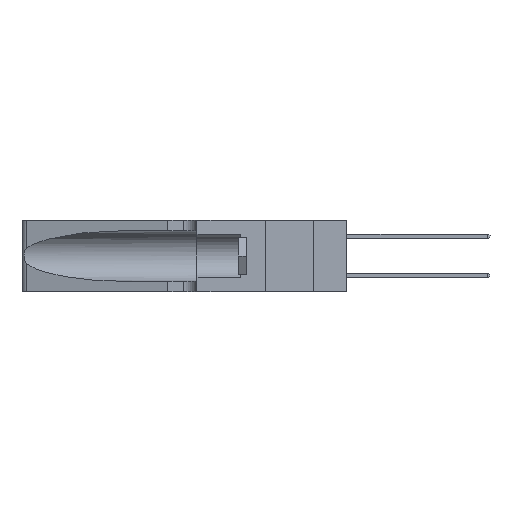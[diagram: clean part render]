
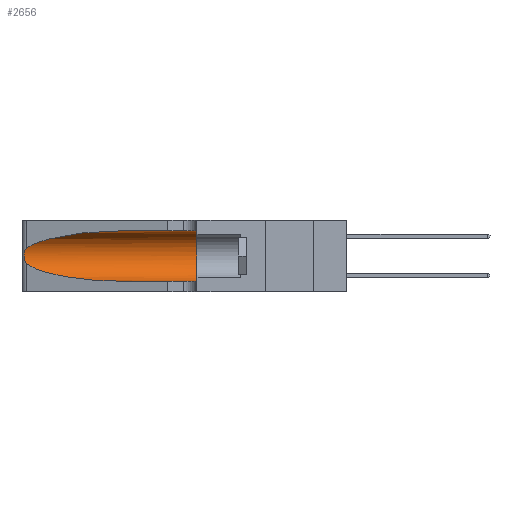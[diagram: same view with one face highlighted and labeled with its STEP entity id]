
A CAD part, left-side view. The second image highlights one B-rep face of the part: STEP entity #2656.
In plain terms, the highlighted cylindrical face has radius 3.308 mm (diameter 6.617 mm), a partial arc.
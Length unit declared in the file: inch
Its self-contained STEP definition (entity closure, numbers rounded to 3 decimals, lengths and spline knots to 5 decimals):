
#344 = VECTOR ( 'NONE', #13298, 39.37008 ) ;
#855 = CIRCLE ( 'NONE', #21152, 0.13025 ) ;
#1330 = DIRECTION ( 'NONE',  ( 0., -1., 0. ) ) ;
#1814 = CARTESIAN_POINT ( 'NONE',  ( 0.1305, 1.61858, 0.05475 ) ) ;
#1860 = DIRECTION ( 'NONE',  ( 0., 1., 0. ) ) ;
#2656 = ADVANCED_FACE ( 'NONE', ( #17979 ), #35239, .F. ) ;
#2858 = VECTOR ( 'NONE', #27332, 39.37008 ) ;
#2972 = VERTEX_POINT ( 'NONE', #34383 ) ;
#3401 = CARTESIAN_POINT ( 'NONE',  ( 0.25487, 1.22718, 0.14631 ) ) ;
#3728 = CARTESIAN_POINT ( 'NONE',  ( 0.18966, 0.96281, 0.31525 ) ) ;
#3752 = CARTESIAN_POINT ( 'NONE',  ( 0.2373, 1.15595, 0.08982 ) ) ;
#4124 = VERTEX_POINT ( 'NONE', #12017 ) ;
#4175 = EDGE_CURVE ( 'NONE', #15163, #4124, #11915, .T. ) ;
#4205 = CARTESIAN_POINT ( 'NONE',  ( 0.25854, 1.2359, 0.20912 ) ) ;
#4450 = ORIENTED_EDGE ( 'NONE', *, *, #34418, .F. ) ;
#6496 = CARTESIAN_POINT ( 'NONE',  ( 0.2373, 1.15595, 0.28018 ) ) ;
#7114 = CARTESIAN_POINT ( 'NONE',  ( 0.18966, 0.96281, 0.05475 ) ) ;
#7706 = EDGE_LOOP ( 'NONE', ( #17933, #35705, #15451, #27042, #4450, #12828 ) ) ;
#7805 = EDGE_CURVE ( 'NONE', #33567, #8279, #21128, .T. ) ;
#8279 = VERTEX_POINT ( 'NONE', #16266 ) ;
#9377 = EDGE_CURVE ( 'NONE', #2972, #33567, #30256, .T. ) ;
#11073 = AXIS2_PLACEMENT_3D ( 'NONE', #20027, #1330, #31758 ) ;
#11915 = LINE ( 'NONE', #25645, #2858 ) ;
#12017 = CARTESIAN_POINT ( 'NONE',  ( 0.1305, 0.35, 0.31525 ) ) ;
#12051 = CARTESIAN_POINT ( 'NONE',  ( 0.26018, 1.23835, 0.19895 ) ) ;
#12190 = CARTESIAN_POINT ( 'NONE',  ( 0.25487, 1.22718, 0.14631 ) ) ;
#12828 = ORIENTED_EDGE ( 'NONE', *, *, #4175, .F. ) ;
#13298 = DIRECTION ( 'NONE',  ( 0., -1., 0. ) ) ;
#13360 = CARTESIAN_POINT ( 'NONE',  ( 0.25555, 1.22993, 0.14849 ) ) ;
#13477 = DIRECTION ( 'NONE',  ( 0., 0., 1. ) ) ;
#14218 = CARTESIAN_POINT ( 'NONE',  ( 0.25487, 1.22718, 0.22369 ) ) ;
#14341 = CARTESIAN_POINT ( 'NONE',  ( 0.25555, 1.22994, 0.2215 ) ) ;
#15117 = EDGE_CURVE ( 'NONE', #15163, #2972, #15892, .T. ) ;
#15163 = VERTEX_POINT ( 'NONE', #28857 ) ;
#15451 = ORIENTED_EDGE ( 'NONE', *, *, #7805, .T. ) ;
#15892 =( BOUNDED_CURVE ( )  B_SPLINE_CURVE ( 3, ( #30749, #3728, #6496, #25653 ),
 .UNSPECIFIED., .F., .F. ) 
 B_SPLINE_CURVE_WITH_KNOTS ( ( 4, 4 ),
 ( 1.5708, 2.84003 ),
 .UNSPECIFIED. ) 
 CURVE ( )  GEOMETRIC_REPRESENTATION_ITEM ( )  RATIONAL_B_SPLINE_CURVE ( ( 1., 0.87, 0.87, 1. ) ) 
 REPRESENTATION_ITEM ( '' )  );
#15898 = CARTESIAN_POINT ( 'NONE',  ( 0.25856, 1.23593, 0.16098 ) ) ;
#16018 = CARTESIAN_POINT ( 'NONE',  ( 0.25639, 1.23186, 0.15144 ) ) ;
#16266 = CARTESIAN_POINT ( 'NONE',  ( 0.1305, 0.72297, 0.05475 ) ) ;
#17693 = CARTESIAN_POINT ( 'NONE',  ( 0.25639, 1.23184, 0.21858 ) ) ;
#17933 = ORIENTED_EDGE ( 'NONE', *, *, #15117, .T. ) ;
#17979 = FACE_OUTER_BOUND ( 'NONE', #7706, .T. ) ;
#18773 = CARTESIAN_POINT ( 'NONE',  ( 0.1305, 0.35, 0.185 ) ) ;
#20027 = CARTESIAN_POINT ( 'NONE',  ( 0.1305, 1.61858, 0.185 ) ) ;
#21128 =( BOUNDED_CURVE ( )  B_SPLINE_CURVE ( 3, ( #3401, #3752, #7114, #29048 ),
 .UNSPECIFIED., .F., .F. ) 
 B_SPLINE_CURVE_WITH_KNOTS ( ( 4, 4 ),
 ( 3.44316, 4.71239 ),
 .UNSPECIFIED. ) 
 CURVE ( )  GEOMETRIC_REPRESENTATION_ITEM ( )  RATIONAL_B_SPLINE_CURVE ( ( 1., 0.87, 0.87, 1. ) ) 
 REPRESENTATION_ITEM ( '' )  );
#21152 = AXIS2_PLACEMENT_3D ( 'NONE', #18773, #1860, #13477 ) ;
#24091 = CARTESIAN_POINT ( 'NONE',  ( 0.26017, 1.23833, 0.17102 ) ) ;
#25645 = CARTESIAN_POINT ( 'NONE',  ( 0.1305, 1.61858, 0.31525 ) ) ;
#25653 = CARTESIAN_POINT ( 'NONE',  ( 0.25487, 1.22718, 0.22369 ) ) ;
#27042 = ORIENTED_EDGE ( 'NONE', *, *, #31643, .T. ) ;
#27215 = CARTESIAN_POINT ( 'NONE',  ( 0.25789, 1.23486, 0.15765 ) ) ;
#27332 = DIRECTION ( 'NONE',  ( 0., -1., 0. ) ) ;
#28551 = CARTESIAN_POINT ( 'NONE',  ( 0.25787, 1.23484, 0.2124 ) ) ;
#28702 = VERTEX_POINT ( 'NONE', #30568 ) ;
#28857 = CARTESIAN_POINT ( 'NONE',  ( 0.1305, 0.72297, 0.31525 ) ) ;
#29048 = CARTESIAN_POINT ( 'NONE',  ( 0.1305, 0.72297, 0.05475 ) ) ;
#29770 = CARTESIAN_POINT ( 'NONE',  ( 0.26075, 1.23896, 0.178 ) ) ;
#30256 = B_SPLINE_CURVE_WITH_KNOTS ( 'NONE', 3,
 ( #14218, #14341, #17693, #28551, #4205, #12051, #31574, #29770, #24091, #15898, #27215, #16018, #13360, #35422 ),
 .UNSPECIFIED., .F., .F.,
 ( 4, 2, 2, 2, 2, 2, 4 ),
 ( 0., 0.00027, 0.00053, 0.00107, 0.0016, 0.00187, 0.00214 ),
 .UNSPECIFIED. ) ;
#30568 = CARTESIAN_POINT ( 'NONE',  ( 0.1305, 0.35, 0.05475 ) ) ;
#30611 = LINE ( 'NONE', #1814, #344 ) ;
#30749 = CARTESIAN_POINT ( 'NONE',  ( 0.1305, 0.72297, 0.31525 ) ) ;
#31574 = CARTESIAN_POINT ( 'NONE',  ( 0.26075, 1.23896, 0.19203 ) ) ;
#31643 = EDGE_CURVE ( 'NONE', #8279, #28702, #30611, .T. ) ;
#31758 = DIRECTION ( 'NONE',  ( 0., 0., -1. ) ) ;
#33567 = VERTEX_POINT ( 'NONE', #12190 ) ;
#34383 = CARTESIAN_POINT ( 'NONE',  ( 0.25487, 1.22718, 0.22369 ) ) ;
#34418 = EDGE_CURVE ( 'NONE', #4124, #28702, #855, .T. ) ;
#35239 = CYLINDRICAL_SURFACE ( 'NONE', #11073, 0.13025 ) ;
#35422 = CARTESIAN_POINT ( 'NONE',  ( 0.25487, 1.22718, 0.14631 ) ) ;
#35705 = ORIENTED_EDGE ( 'NONE', *, *, #9377, .T. ) ;
